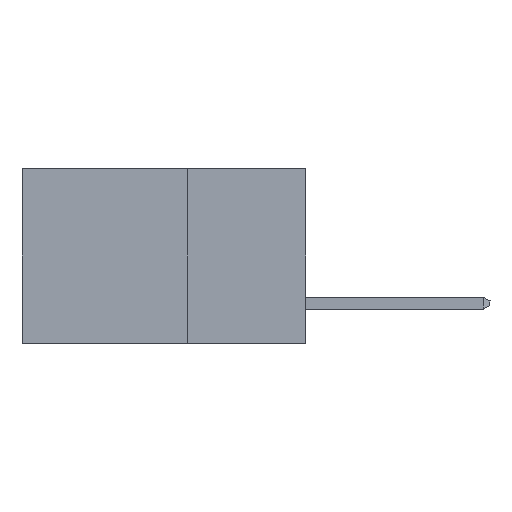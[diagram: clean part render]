
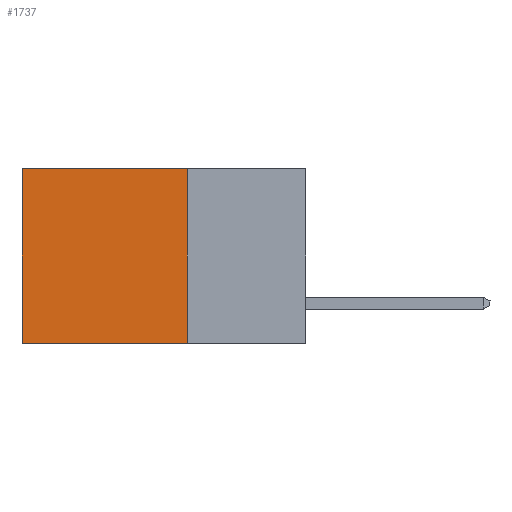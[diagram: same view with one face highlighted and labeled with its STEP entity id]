
A CAD part, left-side view. The second image highlights one B-rep face of the part: STEP entity #1737.
In plain terms, the highlighted planar face has unit normal (-1, 0, 0).
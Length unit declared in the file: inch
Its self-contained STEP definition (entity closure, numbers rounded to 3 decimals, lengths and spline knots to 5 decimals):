
#383 = DIRECTION ( 'NONE',  ( 1., 0., 0. ) ) ;
#1133 = AXIS2_PLACEMENT_3D ( 'NONE', #17114, #383, #17320 ) ;
#1737 = ADVANCED_FACE ( 'NONE', ( #16346 ), #7585, .F. ) ;
#4392 = DIRECTION ( 'NONE',  ( 0., 1., 0. ) ) ;
#5725 = DIRECTION ( 'NONE',  ( 0., 0., -1. ) ) ;
#5763 = EDGE_CURVE ( 'NONE', #9632, #23713, #25758, .T. ) ;
#7080 = EDGE_CURVE ( 'NONE', #9253, #23713, #18971, .T. ) ;
#7585 = PLANE ( 'NONE',  #1133 ) ;
#7894 = EDGE_LOOP ( 'NONE', ( #24394, #13514, #28183, #10629 ) ) ;
#9253 = VERTEX_POINT ( 'NONE', #14866 ) ;
#9632 = VERTEX_POINT ( 'NONE', #18735 ) ;
#10071 = VECTOR ( 'NONE', #18764, 39.37008 ) ;
#10629 = ORIENTED_EDGE ( 'NONE', *, *, #21273, .T. ) ;
#11130 = VECTOR ( 'NONE', #5725, 39.37008 ) ;
#12399 = CARTESIAN_POINT ( 'NONE',  ( 0.298, 0.25, 0. ) ) ;
#12953 = CARTESIAN_POINT ( 'NONE',  ( 0.298, 0.25, 0. ) ) ;
#13514 = ORIENTED_EDGE ( 'NONE', *, *, #5763, .F. ) ;
#14866 = CARTESIAN_POINT ( 'NONE',  ( 0.298, 0.6, 0. ) ) ;
#15250 = CARTESIAN_POINT ( 'NONE',  ( 0.298, 0.6, -0.37 ) ) ;
#16346 = FACE_OUTER_BOUND ( 'NONE', #7894, .T. ) ;
#16555 = LINE ( 'NONE', #28280, #10071 ) ;
#17114 = CARTESIAN_POINT ( 'NONE',  ( 0.298, 0.25, 0. ) ) ;
#17151 = EDGE_CURVE ( 'NONE', #19885, #9632, #24664, .T. ) ;
#17320 = DIRECTION ( 'NONE',  ( 0., 0., -1. ) ) ;
#18735 = CARTESIAN_POINT ( 'NONE',  ( 0.298, 0.25, -0.37 ) ) ;
#18764 = DIRECTION ( 'NONE',  ( 0., 1., 0. ) ) ;
#18971 = LINE ( 'NONE', #23887, #24570 ) ;
#19372 = VECTOR ( 'NONE', #4392, 39.37008 ) ;
#19885 = VERTEX_POINT ( 'NONE', #12399 ) ;
#21273 = EDGE_CURVE ( 'NONE', #19885, #9253, #16555, .T. ) ;
#23559 = CARTESIAN_POINT ( 'NONE',  ( 0.298, 0.25, -0.37 ) ) ;
#23713 = VERTEX_POINT ( 'NONE', #15250 ) ;
#23887 = CARTESIAN_POINT ( 'NONE',  ( 0.298, 0.6, 0. ) ) ;
#24394 = ORIENTED_EDGE ( 'NONE', *, *, #7080, .T. ) ;
#24570 = VECTOR ( 'NONE', #31112, 39.37008 ) ;
#24664 = LINE ( 'NONE', #12953, #11130 ) ;
#25758 = LINE ( 'NONE', #23559, #19372 ) ;
#28183 = ORIENTED_EDGE ( 'NONE', *, *, #17151, .F. ) ;
#28280 = CARTESIAN_POINT ( 'NONE',  ( 0.298, 0.25, 0. ) ) ;
#31112 = DIRECTION ( 'NONE',  ( 0., 0., -1. ) ) ;
